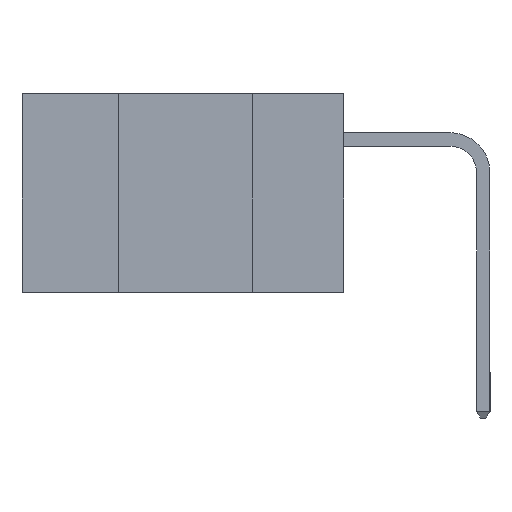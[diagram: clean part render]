
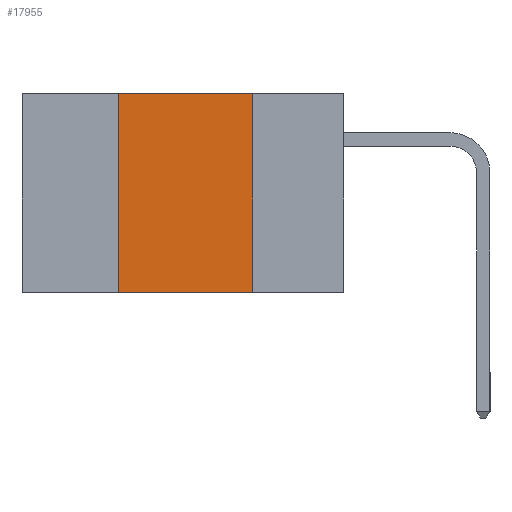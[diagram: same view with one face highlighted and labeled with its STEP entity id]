
A CAD part, left-side view. The second image highlights one B-rep face of the part: STEP entity #17955.
In plain terms, the highlighted planar face has unit normal (-1, 0, 0).
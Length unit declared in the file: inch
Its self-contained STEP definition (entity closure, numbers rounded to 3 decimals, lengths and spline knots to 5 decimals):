
#463 = PLANE ( 'NONE',  #9988 ) ;
#617 = EDGE_CURVE ( 'NONE', #16167, #18327, #12632, .T. ) ;
#812 = ORIENTED_EDGE ( 'NONE', *, *, #11116, .T. ) ;
#3708 = EDGE_LOOP ( 'NONE', ( #9065, #18795, #6384, #812 ) ) ;
#4687 = DIRECTION ( 'NONE',  ( 0., 0., -1. ) ) ;
#5237 = DIRECTION ( 'NONE',  ( 0., -1., 0. ) ) ;
#5251 = CARTESIAN_POINT ( 'NONE',  ( 0., 0.17, 0. ) ) ;
#5321 = FACE_OUTER_BOUND ( 'NONE', #3708, .T. ) ;
#5513 = VERTEX_POINT ( 'NONE', #10398 ) ;
#6384 = ORIENTED_EDGE ( 'NONE', *, *, #617, .F. ) ;
#6830 = CARTESIAN_POINT ( 'NONE',  ( 0., 0.42, 0. ) ) ;
#7365 = VECTOR ( 'NONE', #5237, 39.37008 ) ;
#8281 = VECTOR ( 'NONE', #16217, 39.37008 ) ;
#8305 = VERTEX_POINT ( 'NONE', #13536 ) ;
#9065 = ORIENTED_EDGE ( 'NONE', *, *, #16948, .F. ) ;
#9988 = AXIS2_PLACEMENT_3D ( 'NONE', #12949, #14063, #4687 ) ;
#10126 = CARTESIAN_POINT ( 'NONE',  ( 0., 0.6, -0.37 ) ) ;
#10398 = CARTESIAN_POINT ( 'NONE',  ( 0., 0.17, -0.37 ) ) ;
#11013 = LINE ( 'NONE', #5251, #8281 ) ;
#11116 = EDGE_CURVE ( 'NONE', #16167, #5513, #12998, .T. ) ;
#11235 = CARTESIAN_POINT ( 'NONE',  ( 0., 0.42, -0.37 ) ) ;
#11517 = LINE ( 'NONE', #17662, #7365 ) ;
#11642 = EDGE_CURVE ( 'NONE', #18327, #8305, #11517, .T. ) ;
#12632 = LINE ( 'NONE', #6830, #17545 ) ;
#12949 = CARTESIAN_POINT ( 'NONE',  ( 0., 0.6, 0. ) ) ;
#12998 = LINE ( 'NONE', #10126, #13258 ) ;
#13004 = DIRECTION ( 'NONE',  ( 0., 0., 1. ) ) ;
#13258 = VECTOR ( 'NONE', #18041, 39.37008 ) ;
#13536 = CARTESIAN_POINT ( 'NONE',  ( 0., 0.17, 0. ) ) ;
#14063 = DIRECTION ( 'NONE',  ( 1., 0., 0. ) ) ;
#16167 = VERTEX_POINT ( 'NONE', #11235 ) ;
#16217 = DIRECTION ( 'NONE',  ( 0., 0., -1. ) ) ;
#16948 = EDGE_CURVE ( 'NONE', #8305, #5513, #11013, .T. ) ;
#17545 = VECTOR ( 'NONE', #13004, 39.37008 ) ;
#17662 = CARTESIAN_POINT ( 'NONE',  ( 0., 0.6, 0. ) ) ;
#17955 = ADVANCED_FACE ( 'NONE', ( #5321 ), #463, .F. ) ;
#18041 = DIRECTION ( 'NONE',  ( 0., -1., 0. ) ) ;
#18327 = VERTEX_POINT ( 'NONE', #19972 ) ;
#18795 = ORIENTED_EDGE ( 'NONE', *, *, #11642, .F. ) ;
#19972 = CARTESIAN_POINT ( 'NONE',  ( 0., 0.42, 0. ) ) ;
